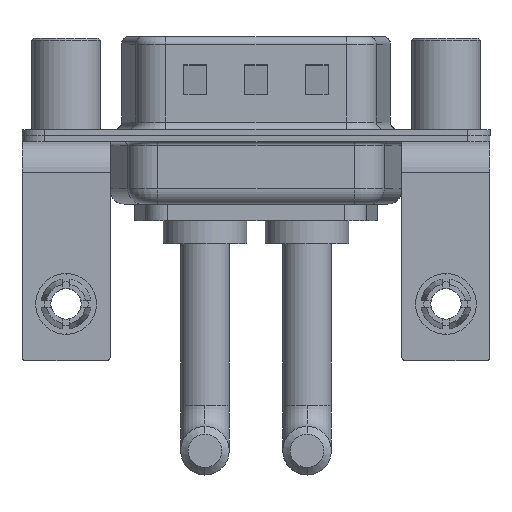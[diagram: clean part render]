
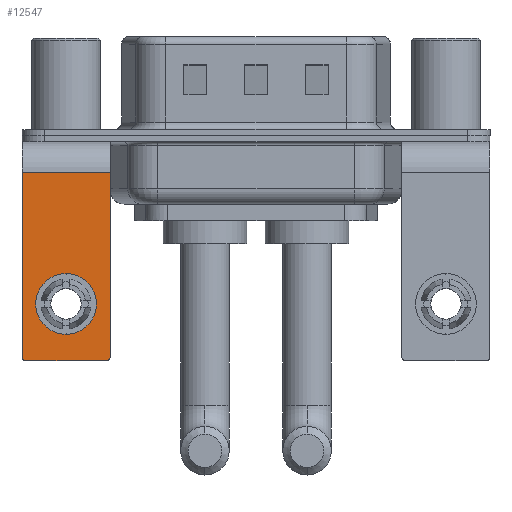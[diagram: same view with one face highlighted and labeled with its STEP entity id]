
A CAD part, front view. The second image highlights one B-rep face of the part: STEP entity #12547.
In plain terms, the highlighted planar face has unit normal (0, -1, 0).
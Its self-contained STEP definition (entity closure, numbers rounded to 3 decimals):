
#321 = AXIS2_PLACEMENT_3D ( 'NONE', #14582, #17481, #2459 ) ;
#527 = VECTOR ( 'NONE', #1420, 1000. ) ;
#535 = EDGE_LOOP ( 'NONE', ( #15442, #12998 ) ) ;
#1420 = DIRECTION ( 'NONE',  ( 0., 0., -1. ) ) ;
#1629 = DIRECTION ( 'NONE',  ( 0., 0., 1. ) ) ;
#1734 = VERTEX_POINT ( 'NONE', #17899 ) ;
#1757 = CARTESIAN_POINT ( 'NONE',  ( 2.9, -6.25, -2.4 ) ) ;
#1980 = DIRECTION ( 'NONE',  ( 0., -1., 0. ) ) ;
#2109 = VERTEX_POINT ( 'NONE', #1757 ) ;
#2200 = LINE ( 'NONE', #7705, #12242 ) ;
#2459 = DIRECTION ( 'NONE',  ( 0., 0., 1. ) ) ;
#3070 = DIRECTION ( 'NONE',  ( 0., 1., 0. ) ) ;
#3336 = DIRECTION ( 'NONE',  ( 0., 0., -1. ) ) ;
#3396 = PLANE ( 'NONE',  #4895 ) ;
#3415 = CARTESIAN_POINT ( 'NONE',  ( -2.9, -6.25, -2.4 ) ) ;
#3563 = DIRECTION ( 'NONE',  ( -1., 0., 0. ) ) ;
#4199 = DIRECTION ( 'NONE',  ( 0., -1., 0. ) ) ;
#4301 = CARTESIAN_POINT ( 'NONE',  ( 2.9, -6.25, -2.4 ) ) ;
#4324 = CARTESIAN_POINT ( 'NONE',  ( 0., -6.25, -11.07 ) ) ;
#4616 = EDGE_CURVE ( 'NONE', #2109, #16395, #13069, .T. ) ;
#4835 = FACE_BOUND ( 'NONE', #535, .T. ) ;
#4895 = AXIS2_PLACEMENT_3D ( 'NONE', #10371, #7922, #5032 ) ;
#4984 = DIRECTION ( 'NONE',  ( -1., 0., 0. ) ) ;
#5032 = DIRECTION ( 'NONE',  ( 0., 0., 1. ) ) ;
#5405 = VERTEX_POINT ( 'NONE', #12598 ) ;
#6145 = LINE ( 'NONE', #3415, #7770 ) ;
#6501 = DIRECTION ( 'NONE',  ( 0., 0., 1. ) ) ;
#6624 = CARTESIAN_POINT ( 'NONE',  ( -2.9, -6.25, -14.55 ) ) ;
#7521 = AXIS2_PLACEMENT_3D ( 'NONE', #9042, #1980, #6501 ) ;
#7705 = CARTESIAN_POINT ( 'NONE',  ( 2.9, -6.25, -14.8 ) ) ;
#7726 = CARTESIAN_POINT ( 'NONE',  ( 0., -6.25, -13.07 ) ) ;
#7770 = VECTOR ( 'NONE', #3336, 1000. ) ;
#7849 = CIRCLE ( 'NONE', #321, 2. ) ;
#7922 = DIRECTION ( 'NONE',  ( 0., 1., 0. ) ) ;
#8114 = LINE ( 'NONE', #4301, #527 ) ;
#8300 = VERTEX_POINT ( 'NONE', #13787 ) ;
#8826 = VERTEX_POINT ( 'NONE', #7726 ) ;
#9042 = CARTESIAN_POINT ( 'NONE',  ( -2.65, -6.25, -14.55 ) ) ;
#9430 = EDGE_CURVE ( 'NONE', #11587, #5405, #2200, .T. ) ;
#9566 = CIRCLE ( 'NONE', #13645, 0.25 ) ;
#9826 = CARTESIAN_POINT ( 'NONE',  ( 2.65, -6.25, -14.55 ) ) ;
#10137 = ORIENTED_EDGE ( 'NONE', *, *, #11450, .F. ) ;
#10371 = CARTESIAN_POINT ( 'NONE',  ( 2.9, -6.25, -2.4 ) ) ;
#10885 = EDGE_CURVE ( 'NONE', #1734, #8826, #17474, .T. ) ;
#11295 = CARTESIAN_POINT ( 'NONE',  ( -2.9, -6.25, -2.4 ) ) ;
#11450 = EDGE_CURVE ( 'NONE', #2109, #8300, #8114, .T. ) ;
#11587 = VERTEX_POINT ( 'NONE', #11968 ) ;
#11710 = AXIS2_PLACEMENT_3D ( 'NONE', #4324, #3070, #1629 ) ;
#11800 = EDGE_CURVE ( 'NONE', #16395, #15755, #6145, .T. ) ;
#11839 = ORIENTED_EDGE ( 'NONE', *, *, #11800, .T. ) ;
#11869 = VECTOR ( 'NONE', #3563, 1000. ) ;
#11968 = CARTESIAN_POINT ( 'NONE',  ( 2.65, -6.25, -14.8 ) ) ;
#12242 = VECTOR ( 'NONE', #4984, 1000. ) ;
#12346 = ORIENTED_EDGE ( 'NONE', *, *, #13240, .T. ) ;
#12547 = ADVANCED_FACE ( 'NONE', ( #4835, #17428 ), #3396, .F. ) ;
#12598 = CARTESIAN_POINT ( 'NONE',  ( -2.65, -6.25, -14.8 ) ) ;
#12816 = DIRECTION ( 'NONE',  ( 0., 0., 1. ) ) ;
#12998 = ORIENTED_EDGE ( 'NONE', *, *, #10885, .T. ) ;
#13069 = LINE ( 'NONE', #17498, #11869 ) ;
#13240 = EDGE_CURVE ( 'NONE', #15755, #5405, #15897, .T. ) ;
#13645 = AXIS2_PLACEMENT_3D ( 'NONE', #9826, #4199, #12816 ) ;
#13787 = CARTESIAN_POINT ( 'NONE',  ( 2.9, -6.25, -14.55 ) ) ;
#14249 = EDGE_CURVE ( 'NONE', #8826, #1734, #7849, .T. ) ;
#14582 = CARTESIAN_POINT ( 'NONE',  ( 0., -6.25, -11.07 ) ) ;
#15057 = EDGE_LOOP ( 'NONE', ( #11839, #12346, #17883, #15177, #10137, #17627 ) ) ;
#15177 = ORIENTED_EDGE ( 'NONE', *, *, #15415, .T. ) ;
#15415 = EDGE_CURVE ( 'NONE', #11587, #8300, #9566, .T. ) ;
#15442 = ORIENTED_EDGE ( 'NONE', *, *, #14249, .T. ) ;
#15755 = VERTEX_POINT ( 'NONE', #6624 ) ;
#15897 = CIRCLE ( 'NONE', #7521, 0.25 ) ;
#16395 = VERTEX_POINT ( 'NONE', #11295 ) ;
#17428 = FACE_OUTER_BOUND ( 'NONE', #15057, .T. ) ;
#17474 = CIRCLE ( 'NONE', #11710, 2. ) ;
#17481 = DIRECTION ( 'NONE',  ( 0., 1., 0. ) ) ;
#17498 = CARTESIAN_POINT ( 'NONE',  ( 2.9, -6.25, -2.4 ) ) ;
#17627 = ORIENTED_EDGE ( 'NONE', *, *, #4616, .T. ) ;
#17883 = ORIENTED_EDGE ( 'NONE', *, *, #9430, .F. ) ;
#17899 = CARTESIAN_POINT ( 'NONE',  ( 0., -6.25, -9.07 ) ) ;
